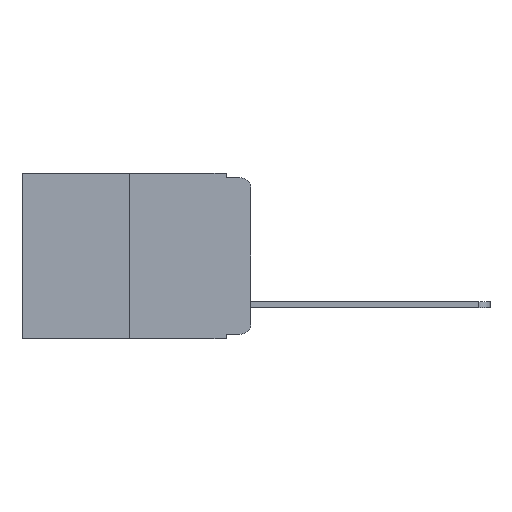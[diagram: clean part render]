
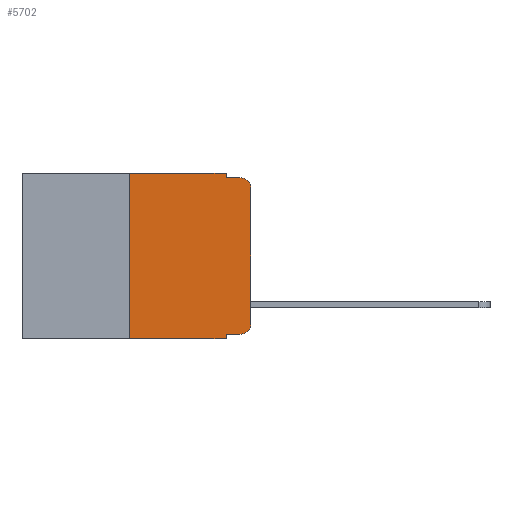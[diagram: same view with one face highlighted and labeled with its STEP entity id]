
A CAD part, left-side view. The second image highlights one B-rep face of the part: STEP entity #5702.
In plain terms, the highlighted planar face has unit normal (-1, 0, 0).
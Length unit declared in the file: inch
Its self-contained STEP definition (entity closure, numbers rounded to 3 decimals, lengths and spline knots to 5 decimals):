
#19 = EDGE_CURVE ( 'NONE', #4457, #6650, #3076, .T. ) ;
#156 = DIRECTION ( 'NONE',  ( 0., -1., 0. ) ) ;
#226 = VECTOR ( 'NONE', #355, 39.37008 ) ;
#355 = DIRECTION ( 'NONE',  ( 0., 0., 1. ) ) ;
#664 = DIRECTION ( 'NONE',  ( 0., 0., -1. ) ) ;
#776 = CARTESIAN_POINT ( 'NONE',  ( 0., 0.473, -0.343 ) ) ;
#791 = ORIENTED_EDGE ( 'NONE', *, *, #7955, .F. ) ;
#952 = DIRECTION ( 'NONE',  ( -1., 0., 0. ) ) ;
#1134 = VERTEX_POINT ( 'NONE', #10076 ) ;
#1308 = CARTESIAN_POINT ( 'NONE',  ( 0., 0.473, 0. ) ) ;
#1635 = EDGE_LOOP ( 'NONE', ( #4647, #2246, #11099, #10791, #5052, #791, #10950, #10692, #11052, #2356 ) ) ;
#1803 = LINE ( 'NONE', #776, #11046 ) ;
#1899 = PLANE ( 'NONE',  #5382 ) ;
#2042 = DIRECTION ( 'NONE',  ( 0., 0., -1. ) ) ;
#2246 = ORIENTED_EDGE ( 'NONE', *, *, #3184, .T. ) ;
#2256 = LINE ( 'NONE', #10825, #6041 ) ;
#2356 = ORIENTED_EDGE ( 'NONE', *, *, #10517, .T. ) ;
#2366 = EDGE_CURVE ( 'NONE', #9616, #5122, #11197, .T. ) ;
#2395 = VERTEX_POINT ( 'NONE', #8279 ) ;
#2399 = CARTESIAN_POINT ( 'NONE',  ( 0., 0., 0. ) ) ;
#2409 = VECTOR ( 'NONE', #2042, 39.37008 ) ;
#2659 = EDGE_CURVE ( 'NONE', #9616, #4356, #3668, .T. ) ;
#2729 = CIRCLE ( 'NONE', #9547, 0.02 ) ;
#2869 = CIRCLE ( 'NONE', #11636, 0.02 ) ;
#3017 = DIRECTION ( 'NONE',  ( 0., 0., -1. ) ) ;
#3076 = LINE ( 'NONE', #4156, #12642 ) ;
#3184 = EDGE_CURVE ( 'NONE', #2395, #6650, #2869, .T. ) ;
#3283 = DIRECTION ( 'NONE',  ( 0., -1., 0. ) ) ;
#3668 = LINE ( 'NONE', #12893, #2409 ) ;
#4156 = CARTESIAN_POINT ( 'NONE',  ( 0., 0.051, -0.01 ) ) ;
#4356 = VERTEX_POINT ( 'NONE', #9749 ) ;
#4457 = VERTEX_POINT ( 'NONE', #9591 ) ;
#4585 = DIRECTION ( 'NONE',  ( -1., 0., 0. ) ) ;
#4647 = ORIENTED_EDGE ( 'NONE', *, *, #11000, .T. ) ;
#4982 = VECTOR ( 'NONE', #12378, 39.37008 ) ;
#5052 = ORIENTED_EDGE ( 'NONE', *, *, #11518, .F. ) ;
#5122 = VERTEX_POINT ( 'NONE', #12003 ) ;
#5259 = FACE_OUTER_BOUND ( 'NONE', #1635, .T. ) ;
#5382 = AXIS2_PLACEMENT_3D ( 'NONE', #11701, #7778, #9774 ) ;
#5695 = EDGE_CURVE ( 'NONE', #12746, #4356, #1803, .T. ) ;
#5702 = ADVANCED_FACE ( 'NONE', ( #5259 ), #1899, .F. ) ;
#6031 = LINE ( 'NONE', #2399, #226 ) ;
#6041 = VECTOR ( 'NONE', #664, 39.37008 ) ;
#6244 = CARTESIAN_POINT ( 'NONE',  ( 0., 0.051, -0.333 ) ) ;
#6324 = CARTESIAN_POINT ( 'NONE',  ( 0., 0.25, 0. ) ) ;
#6351 = CARTESIAN_POINT ( 'NONE',  ( 0., 0.02, -0.01 ) ) ;
#6604 = VERTEX_POINT ( 'NONE', #7396 ) ;
#6643 = CARTESIAN_POINT ( 'NONE',  ( 0., 0.02, -0.313 ) ) ;
#6650 = VERTEX_POINT ( 'NONE', #6351 ) ;
#6676 = CARTESIAN_POINT ( 'NONE',  ( 0., 0.051, -0.333 ) ) ;
#7396 = CARTESIAN_POINT ( 'NONE',  ( 0., 0., -0.313 ) ) ;
#7659 = LINE ( 'NONE', #6324, #4982 ) ;
#7778 = DIRECTION ( 'NONE',  ( 1., 0., 0. ) ) ;
#7955 = EDGE_CURVE ( 'NONE', #12746, #1134, #7659, .T. ) ;
#8279 = CARTESIAN_POINT ( 'NONE',  ( 0., 0., -0.03 ) ) ;
#8306 = DIRECTION ( 'NONE',  ( 0., -1., 0. ) ) ;
#8977 = CARTESIAN_POINT ( 'NONE',  ( 0., 0.02, -0.03 ) ) ;
#9400 = VERTEX_POINT ( 'NONE', #11946 ) ;
#9547 = AXIS2_PLACEMENT_3D ( 'NONE', #6643, #4585, #10696 ) ;
#9591 = CARTESIAN_POINT ( 'NONE',  ( 0., 0.051, -0.01 ) ) ;
#9616 = VERTEX_POINT ( 'NONE', #6244 ) ;
#9749 = CARTESIAN_POINT ( 'NONE',  ( 0., 0.051, -0.343 ) ) ;
#9774 = DIRECTION ( 'NONE',  ( 0., 0., -1. ) ) ;
#9860 = EDGE_CURVE ( 'NONE', #9400, #4457, #2256, .T. ) ;
#10064 = VECTOR ( 'NONE', #8306, 39.37008 ) ;
#10076 = CARTESIAN_POINT ( 'NONE',  ( 0., 0.25, 0. ) ) ;
#10517 = EDGE_CURVE ( 'NONE', #5122, #6604, #2729, .T. ) ;
#10578 = VECTOR ( 'NONE', #3283, 39.37008 ) ;
#10692 = ORIENTED_EDGE ( 'NONE', *, *, #2659, .F. ) ;
#10696 = DIRECTION ( 'NONE',  ( 0., 0., -1. ) ) ;
#10791 = ORIENTED_EDGE ( 'NONE', *, *, #9860, .F. ) ;
#10825 = CARTESIAN_POINT ( 'NONE',  ( 0., 0.051, 0. ) ) ;
#10950 = ORIENTED_EDGE ( 'NONE', *, *, #5695, .T. ) ;
#11000 = EDGE_CURVE ( 'NONE', #6604, #2395, #6031, .T. ) ;
#11014 = LINE ( 'NONE', #1308, #10064 ) ;
#11046 = VECTOR ( 'NONE', #11865, 39.37008 ) ;
#11052 = ORIENTED_EDGE ( 'NONE', *, *, #2366, .T. ) ;
#11099 = ORIENTED_EDGE ( 'NONE', *, *, #19, .F. ) ;
#11197 = LINE ( 'NONE', #6676, #10578 ) ;
#11254 = CARTESIAN_POINT ( 'NONE',  ( 0., 0.25, -0.343 ) ) ;
#11518 = EDGE_CURVE ( 'NONE', #1134, #9400, #11014, .T. ) ;
#11636 = AXIS2_PLACEMENT_3D ( 'NONE', #8977, #952, #3017 ) ;
#11701 = CARTESIAN_POINT ( 'NONE',  ( 0., 0.473, 0. ) ) ;
#11865 = DIRECTION ( 'NONE',  ( 0., -1., 0. ) ) ;
#11946 = CARTESIAN_POINT ( 'NONE',  ( 0., 0.051, 0. ) ) ;
#12003 = CARTESIAN_POINT ( 'NONE',  ( 0., 0.02, -0.333 ) ) ;
#12378 = DIRECTION ( 'NONE',  ( 0., 0., 1. ) ) ;
#12642 = VECTOR ( 'NONE', #156, 39.37008 ) ;
#12746 = VERTEX_POINT ( 'NONE', #11254 ) ;
#12893 = CARTESIAN_POINT ( 'NONE',  ( 0., 0.051, 0. ) ) ;
